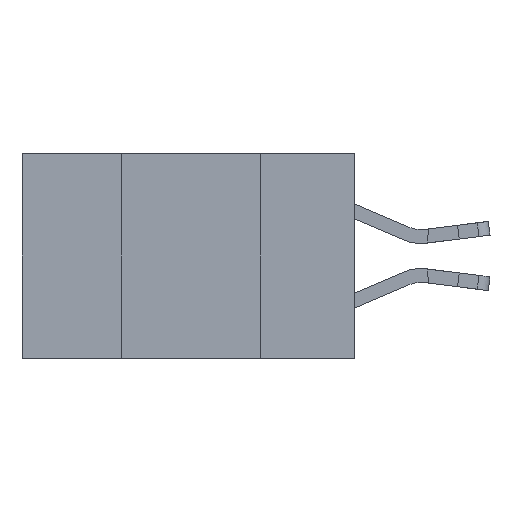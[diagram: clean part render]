
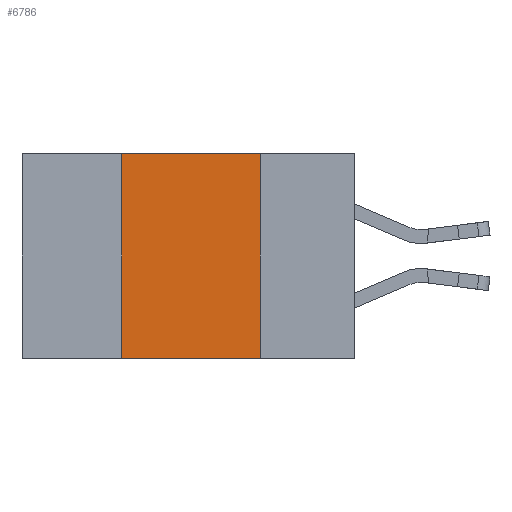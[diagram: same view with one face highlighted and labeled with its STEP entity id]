
A CAD part, left-side view. The second image highlights one B-rep face of the part: STEP entity #6786.
In plain terms, the highlighted planar face has unit normal (-1, 0, 0).
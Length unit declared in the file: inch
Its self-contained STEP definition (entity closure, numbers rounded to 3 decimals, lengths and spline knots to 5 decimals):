
#133 = DIRECTION ( 'NONE',  ( 0., 0., -1. ) ) ;
#143 = EDGE_CURVE ( 'NONE', #6469, #4893, #8742, .T. ) ;
#271 = VERTEX_POINT ( 'NONE', #11410 ) ;
#400 = CARTESIAN_POINT ( 'NONE',  ( 0., 0.6, -0.37 ) ) ;
#1186 = CARTESIAN_POINT ( 'NONE',  ( 0., 0.6, 0. ) ) ;
#1310 = DIRECTION ( 'NONE',  ( 0., 0., 1. ) ) ;
#1366 = DIRECTION ( 'NONE',  ( 0., -1., 0. ) ) ;
#1507 = VECTOR ( 'NONE', #1310, 39.37008 ) ;
#1579 = EDGE_CURVE ( 'NONE', #4893, #12768, #8670, .T. ) ;
#2024 = ORIENTED_EDGE ( 'NONE', *, *, #2506, .T. ) ;
#2506 = EDGE_CURVE ( 'NONE', #6469, #271, #10949, .T. ) ;
#3098 = CARTESIAN_POINT ( 'NONE',  ( 0., 0.42, 0. ) ) ;
#3238 = VECTOR ( 'NONE', #133, 39.37008 ) ;
#3536 = DIRECTION ( 'NONE',  ( 0., -1., 0. ) ) ;
#4386 = CARTESIAN_POINT ( 'NONE',  ( 0., 0.42, 0. ) ) ;
#4893 = VERTEX_POINT ( 'NONE', #3098 ) ;
#5206 = CARTESIAN_POINT ( 'NONE',  ( 0., 0.6, 0. ) ) ;
#5395 = CARTESIAN_POINT ( 'NONE',  ( 0., 0.42, -0.37 ) ) ;
#6308 = AXIS2_PLACEMENT_3D ( 'NONE', #5206, #15295, #12608 ) ;
#6469 = VERTEX_POINT ( 'NONE', #5395 ) ;
#6786 = ADVANCED_FACE ( 'NONE', ( #9693 ), #9905, .F. ) ;
#6889 = LINE ( 'NONE', #16375, #3238 ) ;
#8670 = LINE ( 'NONE', #1186, #11817 ) ;
#8742 = LINE ( 'NONE', #4386, #1507 ) ;
#9693 = FACE_OUTER_BOUND ( 'NONE', #16148, .T. ) ;
#9905 = PLANE ( 'NONE',  #6308 ) ;
#10949 = LINE ( 'NONE', #400, #15374 ) ;
#11244 = CARTESIAN_POINT ( 'NONE',  ( 0., 0.17, 0. ) ) ;
#11410 = CARTESIAN_POINT ( 'NONE',  ( 0., 0.17, -0.37 ) ) ;
#11817 = VECTOR ( 'NONE', #3536, 39.37008 ) ;
#12608 = DIRECTION ( 'NONE',  ( 0., 0., -1. ) ) ;
#12768 = VERTEX_POINT ( 'NONE', #11244 ) ;
#13300 = EDGE_CURVE ( 'NONE', #12768, #271, #6889, .T. ) ;
#13608 = ORIENTED_EDGE ( 'NONE', *, *, #1579, .F. ) ;
#15295 = DIRECTION ( 'NONE',  ( 1., 0., 0. ) ) ;
#15374 = VECTOR ( 'NONE', #1366, 39.37008 ) ;
#16148 = EDGE_LOOP ( 'NONE', ( #16558, #13608, #16256, #2024 ) ) ;
#16256 = ORIENTED_EDGE ( 'NONE', *, *, #143, .F. ) ;
#16375 = CARTESIAN_POINT ( 'NONE',  ( 0., 0.17, 0. ) ) ;
#16558 = ORIENTED_EDGE ( 'NONE', *, *, #13300, .F. ) ;
